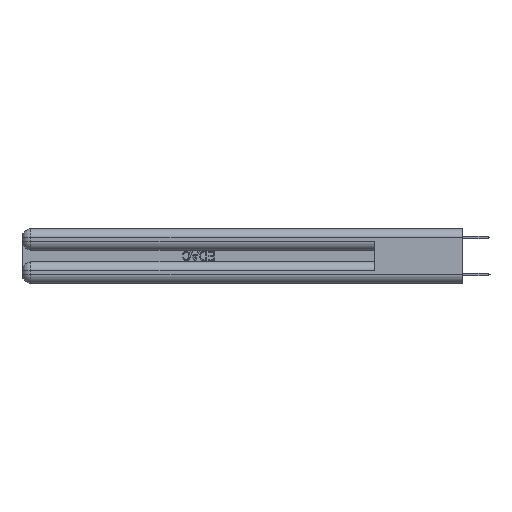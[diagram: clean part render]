
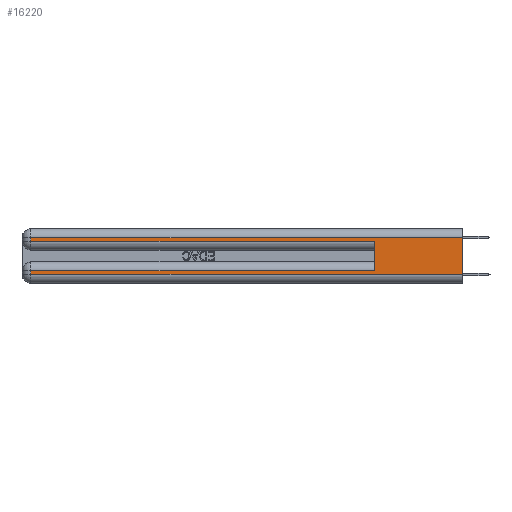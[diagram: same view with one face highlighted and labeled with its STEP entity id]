
A CAD part, left-side view. The second image highlights one B-rep face of the part: STEP entity #16220.
In plain terms, the highlighted planar face has unit normal (-1, 0, 0).
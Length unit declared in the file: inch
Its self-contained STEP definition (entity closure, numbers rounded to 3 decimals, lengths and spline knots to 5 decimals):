
#459 = DIRECTION ( 'NONE',  ( 0., 0., -1. ) ) ;
#1468 = VERTEX_POINT ( 'NONE', #12720 ) ;
#2828 = LINE ( 'NONE', #28758, #24143 ) ;
#3811 = DIRECTION ( 'NONE',  ( 1., 0., 0. ) ) ;
#4344 = VERTEX_POINT ( 'NONE', #29929 ) ;
#4674 = CARTESIAN_POINT ( 'NONE',  ( 0., 2.94, 0.06 ) ) ;
#4733 = LINE ( 'NONE', #17560, #10792 ) ;
#4936 = CARTESIAN_POINT ( 'NONE',  ( 0., 0.6, 0.085 ) ) ;
#5175 = DIRECTION ( 'NONE',  ( 0., 0., -1. ) ) ;
#5972 = CARTESIAN_POINT ( 'NONE',  ( 0., 2.94, 0.37 ) ) ;
#6208 = CARTESIAN_POINT ( 'NONE',  ( 0., 0., 0.31 ) ) ;
#6512 = CARTESIAN_POINT ( 'NONE',  ( 0., 0., 0.285 ) ) ;
#7044 = FACE_OUTER_BOUND ( 'NONE', #24102, .T. ) ;
#7160 = VERTEX_POINT ( 'NONE', #22924 ) ;
#7297 = EDGE_CURVE ( 'NONE', #1468, #7160, #14316, .T. ) ;
#7550 = CARTESIAN_POINT ( 'NONE',  ( 0., 0., 0.37 ) ) ;
#7618 = LINE ( 'NONE', #11997, #22500 ) ;
#7886 = CARTESIAN_POINT ( 'NONE',  ( 0., 2.94, 0.37 ) ) ;
#8194 = ORIENTED_EDGE ( 'NONE', *, *, #31365, .T. ) ;
#8567 = VECTOR ( 'NONE', #5175, 39.37008 ) ;
#9970 = DIRECTION ( 'NONE',  ( 0., -1., 0. ) ) ;
#10196 = VECTOR ( 'NONE', #24170, 39.37008 ) ;
#10792 = VECTOR ( 'NONE', #9970, 39.37008 ) ;
#11612 = VERTEX_POINT ( 'NONE', #4936 ) ;
#11997 = CARTESIAN_POINT ( 'NONE',  ( 0., 0., 0.085 ) ) ;
#12086 = ORIENTED_EDGE ( 'NONE', *, *, #28776, .T. ) ;
#12168 = LINE ( 'NONE', #6208, #10196 ) ;
#12250 = VERTEX_POINT ( 'NONE', #31474 ) ;
#12720 = CARTESIAN_POINT ( 'NONE',  ( 0., 2.94, 0.285 ) ) ;
#13358 = DIRECTION ( 'NONE',  ( 0., 0., 1. ) ) ;
#13673 = VERTEX_POINT ( 'NONE', #4674 ) ;
#14316 = LINE ( 'NONE', #6512, #23558 ) ;
#16220 = ADVANCED_FACE ( 'NONE', ( #7044 ), #32553, .F. ) ;
#16984 = LINE ( 'NONE', #5972, #23016 ) ;
#17560 = CARTESIAN_POINT ( 'NONE',  ( 0., 0., 0.06 ) ) ;
#19137 = AXIS2_PLACEMENT_3D ( 'NONE', #19195, #3811, #21781 ) ;
#19195 = CARTESIAN_POINT ( 'NONE',  ( 0., 0., 0.37 ) ) ;
#20887 = ORIENTED_EDGE ( 'NONE', *, *, #25922, .T. ) ;
#21155 = EDGE_CURVE ( 'NONE', #22196, #12250, #24357, .T. ) ;
#21781 = DIRECTION ( 'NONE',  ( 0., 0., -1. ) ) ;
#21877 = DIRECTION ( 'NONE',  ( 0., 1., 0. ) ) ;
#22196 = VERTEX_POINT ( 'NONE', #32630 ) ;
#22500 = VECTOR ( 'NONE', #21877, 39.37008 ) ;
#22810 = DIRECTION ( 'NONE',  ( 0., 0., -1. ) ) ;
#22920 = EDGE_CURVE ( 'NONE', #31176, #1468, #29437, .T. ) ;
#22924 = CARTESIAN_POINT ( 'NONE',  ( 0., 0.6, 0.285 ) ) ;
#23016 = VECTOR ( 'NONE', #459, 39.37008 ) ;
#23558 = VECTOR ( 'NONE', #32011, 39.37008 ) ;
#23716 = ORIENTED_EDGE ( 'NONE', *, *, #7297, .T. ) ;
#24102 = EDGE_LOOP ( 'NONE', ( #25099, #28231, #26624, #23716, #24475, #20887, #8194, #12086 ) ) ;
#24143 = VECTOR ( 'NONE', #13358, 39.37008 ) ;
#24170 = DIRECTION ( 'NONE',  ( 0., 1., 0. ) ) ;
#24357 = LINE ( 'NONE', #7550, #31164 ) ;
#24475 = ORIENTED_EDGE ( 'NONE', *, *, #25025, .F. ) ;
#25025 = EDGE_CURVE ( 'NONE', #11612, #7160, #2828, .T. ) ;
#25099 = ORIENTED_EDGE ( 'NONE', *, *, #21155, .F. ) ;
#25922 = EDGE_CURVE ( 'NONE', #11612, #4344, #7618, .T. ) ;
#26624 = ORIENTED_EDGE ( 'NONE', *, *, #22920, .T. ) ;
#28231 = ORIENTED_EDGE ( 'NONE', *, *, #31521, .T. ) ;
#28453 = CARTESIAN_POINT ( 'NONE',  ( 0., 2.94, 0.31 ) ) ;
#28758 = CARTESIAN_POINT ( 'NONE',  ( 0., 0.6, 0.145 ) ) ;
#28776 = EDGE_CURVE ( 'NONE', #13673, #12250, #4733, .T. ) ;
#29437 = LINE ( 'NONE', #7886, #8567 ) ;
#29929 = CARTESIAN_POINT ( 'NONE',  ( 0., 2.94, 0.085 ) ) ;
#31164 = VECTOR ( 'NONE', #22810, 39.37008 ) ;
#31176 = VERTEX_POINT ( 'NONE', #28453 ) ;
#31365 = EDGE_CURVE ( 'NONE', #4344, #13673, #16984, .T. ) ;
#31474 = CARTESIAN_POINT ( 'NONE',  ( 0., 0., 0.06 ) ) ;
#31521 = EDGE_CURVE ( 'NONE', #22196, #31176, #12168, .T. ) ;
#32011 = DIRECTION ( 'NONE',  ( 0., -1., 0. ) ) ;
#32553 = PLANE ( 'NONE',  #19137 ) ;
#32630 = CARTESIAN_POINT ( 'NONE',  ( 0., 0., 0.31 ) ) ;
